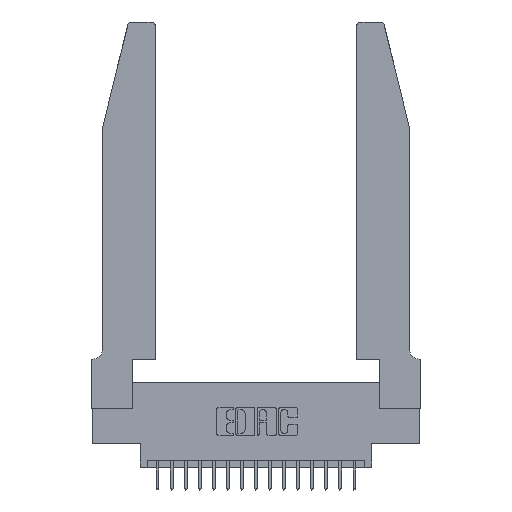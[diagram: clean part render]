
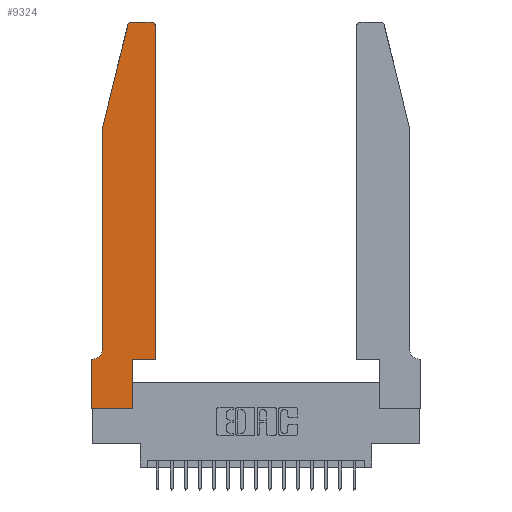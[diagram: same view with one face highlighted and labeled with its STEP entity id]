
A CAD part, top view. The second image highlights one B-rep face of the part: STEP entity #9324.
In plain terms, the highlighted planar face has unit normal (0, 0, 1).
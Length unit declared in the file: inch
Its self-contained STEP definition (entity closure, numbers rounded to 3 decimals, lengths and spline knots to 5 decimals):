
#281 = ORIENTED_EDGE ( 'NONE', *, *, #15180, .T. ) ;
#305 = AXIS2_PLACEMENT_3D ( 'NONE', #9303, #9172, #2784 ) ;
#368 = VERTEX_POINT ( 'NONE', #7876 ) ;
#498 = AXIS2_PLACEMENT_3D ( 'NONE', #17659, #4947, #15955 ) ;
#706 = CARTESIAN_POINT ( 'NONE',  ( 0.2865, 0., 0.37 ) ) ;
#880 = VERTEX_POINT ( 'NONE', #19539 ) ;
#1094 = VECTOR ( 'NONE', #9218, 39.37008 ) ;
#1100 = ORIENTED_EDGE ( 'NONE', *, *, #5554, .T. ) ;
#1184 = DIRECTION ( 'NONE',  ( 0., 0., 1. ) ) ;
#1214 = EDGE_CURVE ( 'NONE', #9928, #10032, #19299, .T. ) ;
#1433 = EDGE_CURVE ( 'NONE', #16051, #880, #13635, .T. ) ;
#1551 = CARTESIAN_POINT ( 'NONE',  ( 0., 0., 0.37 ) ) ;
#1560 = VERTEX_POINT ( 'NONE', #9688 ) ;
#1566 = CARTESIAN_POINT ( 'NONE',  ( 0.0755, 2., 0.37 ) ) ;
#2512 = DIRECTION ( 'NONE',  ( 0., 0., 1. ) ) ;
#2784 = DIRECTION ( 'NONE',  ( -1., 0., 0. ) ) ;
#3669 = CIRCLE ( 'NONE', #305, 0.07 ) ;
#3832 = VERTEX_POINT ( 'NONE', #1551 ) ;
#3890 = EDGE_CURVE ( 'NONE', #368, #17903, #9359, .T. ) ;
#3908 = VERTEX_POINT ( 'NONE', #18937 ) ;
#4238 = CARTESIAN_POINT ( 'NONE',  ( 0.2865, 0.35, 0.37 ) ) ;
#4245 = CARTESIAN_POINT ( 'NONE',  ( 0.0055, 0.35, 0.37 ) ) ;
#4295 = LINE ( 'NONE', #12542, #11904 ) ;
#4947 = DIRECTION ( 'NONE',  ( 0., 0., 1. ) ) ;
#5105 = ORIENTED_EDGE ( 'NONE', *, *, #1214, .T. ) ;
#5554 = EDGE_CURVE ( 'NONE', #880, #3832, #10340, .T. ) ;
#5856 = DIRECTION ( 'NONE',  ( 1., 0., 0. ) ) ;
#6039 = ORIENTED_EDGE ( 'NONE', *, *, #10234, .T. ) ;
#6215 = DIRECTION ( 'NONE',  ( -0.239, -0.971, 0. ) ) ;
#6598 = EDGE_CURVE ( 'NONE', #7194, #9928, #17203, .T. ) ;
#7082 = CARTESIAN_POINT ( 'NONE',  ( 0.4505, 0.35, 0.37 ) ) ;
#7194 = VERTEX_POINT ( 'NONE', #706 ) ;
#7290 = CARTESIAN_POINT ( 'NONE',  ( 0., 0.35, 0.37 ) ) ;
#7876 = CARTESIAN_POINT ( 'NONE',  ( 0.25487, 2.72718, 0.37 ) ) ;
#7908 = ORIENTED_EDGE ( 'NONE', *, *, #1433, .T. ) ;
#8569 = DIRECTION ( 'NONE',  ( -1., 0., 0. ) ) ;
#8949 = PLANE ( 'NONE',  #14467 ) ;
#9172 = DIRECTION ( 'NONE',  ( 0., 0., -1. ) ) ;
#9218 = DIRECTION ( 'NONE',  ( -1., 0., 0. ) ) ;
#9248 = CIRCLE ( 'NONE', #498, 0.03 ) ;
#9303 = CARTESIAN_POINT ( 'NONE',  ( 0.0055, 0.42, 0.37 ) ) ;
#9324 = ADVANCED_FACE ( 'NONE', ( #18808 ), #8949, .T. ) ;
#9359 = LINE ( 'NONE', #9456, #18707 ) ;
#9456 = CARTESIAN_POINT ( 'NONE',  ( 0.0755, 2., 0.37 ) ) ;
#9688 = CARTESIAN_POINT ( 'NONE',  ( 0.4505, 2.72, 0.37 ) ) ;
#9928 = VERTEX_POINT ( 'NONE', #20198 ) ;
#9975 = VECTOR ( 'NONE', #18080, 39.37008 ) ;
#10032 = VERTEX_POINT ( 'NONE', #20337 ) ;
#10190 = CARTESIAN_POINT ( 'NONE',  ( 0.4505, 0.35, 0.37 ) ) ;
#10234 = EDGE_CURVE ( 'NONE', #17903, #16780, #14358, .T. ) ;
#10340 = LINE ( 'NONE', #15025, #13810 ) ;
#10350 = CARTESIAN_POINT ( 'NONE',  ( 0.2605, 2.75, 0.37 ) ) ;
#10721 = ORIENTED_EDGE ( 'NONE', *, *, #12457, .T. ) ;
#11523 = EDGE_CURVE ( 'NONE', #1560, #14565, #9248, .T. ) ;
#11904 = VECTOR ( 'NONE', #18777, 39.37008 ) ;
#12027 = EDGE_CURVE ( 'NONE', #10032, #1560, #14170, .T. ) ;
#12296 = DIRECTION ( 'NONE',  ( 0., 1., 0. ) ) ;
#12457 = EDGE_CURVE ( 'NONE', #3832, #7194, #4295, .T. ) ;
#12542 = CARTESIAN_POINT ( 'NONE',  ( 0., 0., 0.37 ) ) ;
#12915 = ORIENTED_EDGE ( 'NONE', *, *, #16617, .T. ) ;
#12975 = CIRCLE ( 'NONE', #17699, 0.03 ) ;
#13023 = VECTOR ( 'NONE', #12296, 39.37008 ) ;
#13201 = LINE ( 'NONE', #10350, #13966 ) ;
#13237 = DIRECTION ( 'NONE',  ( 0., -1., 0. ) ) ;
#13357 = CARTESIAN_POINT ( 'NONE',  ( 0.284, 2.72, 0.37 ) ) ;
#13599 = EDGE_LOOP ( 'NONE', ( #19673, #12915, #16096, #6039, #281, #7908, #1100, #10721, #16755, #5105, #19803, #14666 ) ) ;
#13635 = LINE ( 'NONE', #18630, #1094 ) ;
#13810 = VECTOR ( 'NONE', #16591, 39.37008 ) ;
#13966 = VECTOR ( 'NONE', #8569, 39.37008 ) ;
#14170 = LINE ( 'NONE', #7082, #9975 ) ;
#14358 = LINE ( 'NONE', #17901, #19750 ) ;
#14467 = AXIS2_PLACEMENT_3D ( 'NONE', #7290, #1184, #5856 ) ;
#14565 = VERTEX_POINT ( 'NONE', #17658 ) ;
#14666 = ORIENTED_EDGE ( 'NONE', *, *, #11523, .T. ) ;
#14937 = DIRECTION ( 'NONE',  ( 1., 0., 0. ) ) ;
#15025 = CARTESIAN_POINT ( 'NONE',  ( 0., 0., 0.37 ) ) ;
#15180 = EDGE_CURVE ( 'NONE', #16780, #16051, #3669, .T. ) ;
#15955 = DIRECTION ( 'NONE',  ( 1., 0., 0. ) ) ;
#16051 = VERTEX_POINT ( 'NONE', #4245 ) ;
#16096 = ORIENTED_EDGE ( 'NONE', *, *, #3890, .T. ) ;
#16454 = DIRECTION ( 'NONE',  ( 1., 0., 0. ) ) ;
#16591 = DIRECTION ( 'NONE',  ( 0., -1., 0. ) ) ;
#16617 = EDGE_CURVE ( 'NONE', #3908, #368, #12975, .T. ) ;
#16755 = ORIENTED_EDGE ( 'NONE', *, *, #6598, .T. ) ;
#16780 = VERTEX_POINT ( 'NONE', #18655 ) ;
#16847 = VECTOR ( 'NONE', #14937, 39.37008 ) ;
#17203 = LINE ( 'NONE', #4238, #13023 ) ;
#17658 = CARTESIAN_POINT ( 'NONE',  ( 0.4205, 2.75, 0.37 ) ) ;
#17659 = CARTESIAN_POINT ( 'NONE',  ( 0.4205, 2.72, 0.37 ) ) ;
#17699 = AXIS2_PLACEMENT_3D ( 'NONE', #13357, #2512, #16454 ) ;
#17901 = CARTESIAN_POINT ( 'NONE',  ( 0.0755, 2., 0.37 ) ) ;
#17903 = VERTEX_POINT ( 'NONE', #1566 ) ;
#18080 = DIRECTION ( 'NONE',  ( 0., 1., 0. ) ) ;
#18630 = CARTESIAN_POINT ( 'NONE',  ( 0.0755, 0.35, 0.37 ) ) ;
#18655 = CARTESIAN_POINT ( 'NONE',  ( 0.0755, 0.42, 0.37 ) ) ;
#18707 = VECTOR ( 'NONE', #6215, 39.37008 ) ;
#18777 = DIRECTION ( 'NONE',  ( 1., 0., 0. ) ) ;
#18808 = FACE_OUTER_BOUND ( 'NONE', #13599, .T. ) ;
#18937 = CARTESIAN_POINT ( 'NONE',  ( 0.284, 2.75, 0.37 ) ) ;
#19299 = LINE ( 'NONE', #10190, #16847 ) ;
#19539 = CARTESIAN_POINT ( 'NONE',  ( 0., 0.35, 0.37 ) ) ;
#19673 = ORIENTED_EDGE ( 'NONE', *, *, #20228, .T. ) ;
#19750 = VECTOR ( 'NONE', #13237, 39.37008 ) ;
#19803 = ORIENTED_EDGE ( 'NONE', *, *, #12027, .T. ) ;
#20198 = CARTESIAN_POINT ( 'NONE',  ( 0.2865, 0.35, 0.37 ) ) ;
#20228 = EDGE_CURVE ( 'NONE', #14565, #3908, #13201, .T. ) ;
#20337 = CARTESIAN_POINT ( 'NONE',  ( 0.4505, 0.35, 0.37 ) ) ;
